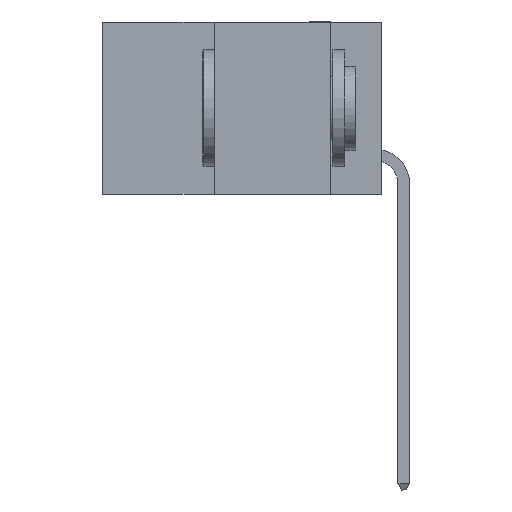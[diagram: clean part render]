
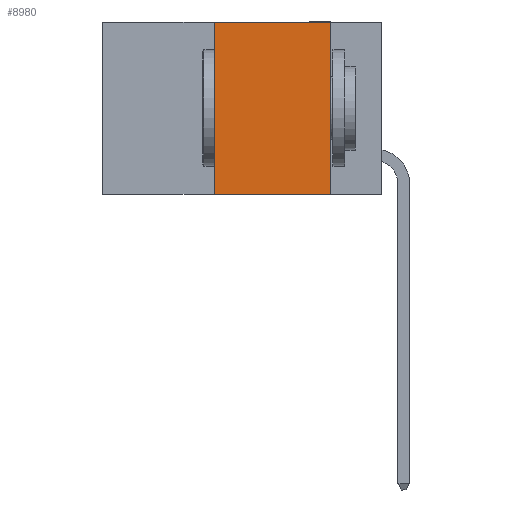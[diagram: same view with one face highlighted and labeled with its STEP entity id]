
A CAD part, left-side view. The second image highlights one B-rep face of the part: STEP entity #8980.
In plain terms, the highlighted planar face has unit normal (-1, 0, 0).
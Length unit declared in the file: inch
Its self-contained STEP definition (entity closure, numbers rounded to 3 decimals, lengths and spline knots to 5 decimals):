
#485 = ORIENTED_EDGE ( 'NONE', *, *, #16486, .F. ) ;
#763 = CARTESIAN_POINT ( 'NONE',  ( 0., 0.6, 0. ) ) ;
#949 = DIRECTION ( 'NONE',  ( 0., 0., -1. ) ) ;
#1592 = CARTESIAN_POINT ( 'NONE',  ( 0., 0.36, 0. ) ) ;
#2172 = CARTESIAN_POINT ( 'NONE',  ( 0., 0.36, -0.37 ) ) ;
#2211 = EDGE_LOOP ( 'NONE', ( #485, #13208, #7529, #15214 ) ) ;
#4150 = LINE ( 'NONE', #16247, #14563 ) ;
#4888 = VECTOR ( 'NONE', #9100, 39.37008 ) ;
#5114 = VECTOR ( 'NONE', #14022, 39.37008 ) ;
#5643 = VERTEX_POINT ( 'NONE', #15661 ) ;
#5806 = LINE ( 'NONE', #1592, #16104 ) ;
#6717 = CARTESIAN_POINT ( 'NONE',  ( 0., 0.11, -0.37 ) ) ;
#7247 = DIRECTION ( 'NONE',  ( 0., 0., 1. ) ) ;
#7529 = ORIENTED_EDGE ( 'NONE', *, *, #11097, .F. ) ;
#8398 = VERTEX_POINT ( 'NONE', #13351 ) ;
#8737 = AXIS2_PLACEMENT_3D ( 'NONE', #763, #9308, #949 ) ;
#8772 = LINE ( 'NONE', #9999, #5114 ) ;
#8941 = VERTEX_POINT ( 'NONE', #2172 ) ;
#8980 = ADVANCED_FACE ( 'NONE', ( #14598 ), #17265, .F. ) ;
#9100 = DIRECTION ( 'NONE',  ( 0., -1., 0. ) ) ;
#9308 = DIRECTION ( 'NONE',  ( 1., 0., 0. ) ) ;
#9384 = LINE ( 'NONE', #13098, #4888 ) ;
#9606 = DIRECTION ( 'NONE',  ( 0., 0., -1. ) ) ;
#9999 = CARTESIAN_POINT ( 'NONE',  ( 0., 0.6, -0.37 ) ) ;
#11097 = EDGE_CURVE ( 'NONE', #8941, #5643, #5806, .T. ) ;
#12874 = EDGE_CURVE ( 'NONE', #8941, #14662, #8772, .T. ) ;
#13080 = EDGE_CURVE ( 'NONE', #5643, #8398, #9384, .T. ) ;
#13098 = CARTESIAN_POINT ( 'NONE',  ( 0., 0.6, 0. ) ) ;
#13208 = ORIENTED_EDGE ( 'NONE', *, *, #13080, .F. ) ;
#13351 = CARTESIAN_POINT ( 'NONE',  ( 0., 0.11, 0. ) ) ;
#14022 = DIRECTION ( 'NONE',  ( 0., -1., 0. ) ) ;
#14563 = VECTOR ( 'NONE', #9606, 39.37008 ) ;
#14598 = FACE_OUTER_BOUND ( 'NONE', #2211, .T. ) ;
#14662 = VERTEX_POINT ( 'NONE', #6717 ) ;
#15214 = ORIENTED_EDGE ( 'NONE', *, *, #12874, .T. ) ;
#15661 = CARTESIAN_POINT ( 'NONE',  ( 0., 0.36, 0. ) ) ;
#16104 = VECTOR ( 'NONE', #7247, 39.37008 ) ;
#16247 = CARTESIAN_POINT ( 'NONE',  ( 0., 0.11, 0. ) ) ;
#16486 = EDGE_CURVE ( 'NONE', #8398, #14662, #4150, .T. ) ;
#17265 = PLANE ( 'NONE',  #8737 ) ;
